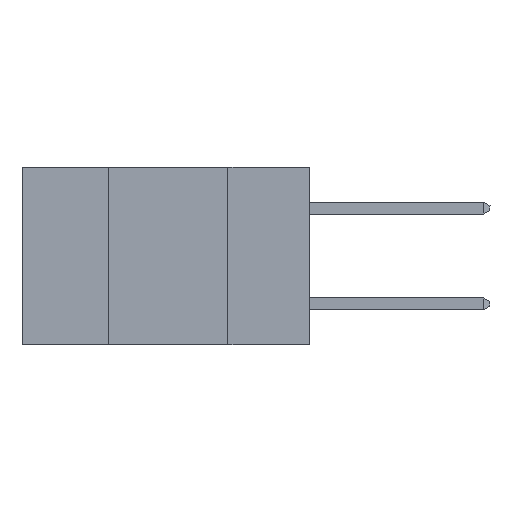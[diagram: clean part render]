
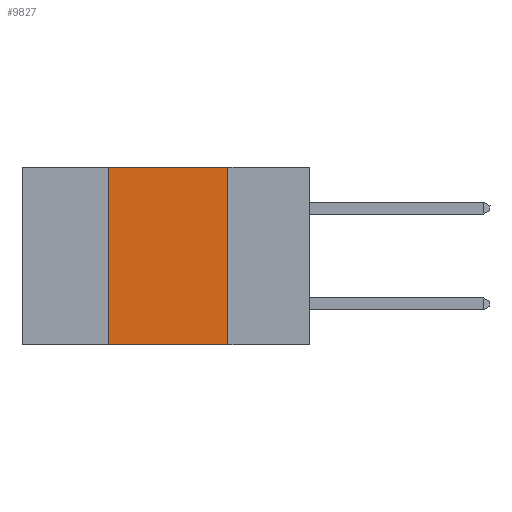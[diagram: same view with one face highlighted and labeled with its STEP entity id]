
A CAD part, left-side view. The second image highlights one B-rep face of the part: STEP entity #9827.
In plain terms, the highlighted planar face has unit normal (-1, 0, 0).
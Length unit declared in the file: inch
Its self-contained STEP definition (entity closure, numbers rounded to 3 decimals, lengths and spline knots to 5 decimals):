
#438 = FACE_OUTER_BOUND ( 'NONE', #6962, .T. ) ;
#467 = ORIENTED_EDGE ( 'NONE', *, *, #2694, .F. ) ;
#896 = CARTESIAN_POINT ( 'NONE',  ( 0., 0.42, 0. ) ) ;
#1671 = DIRECTION ( 'NONE',  ( 1., 0., 0. ) ) ;
#1912 = CARTESIAN_POINT ( 'NONE',  ( 0., 0.42, -0.37 ) ) ;
#2023 = VECTOR ( 'NONE', #8793, 39.37008 ) ;
#2311 = VERTEX_POINT ( 'NONE', #13477 ) ;
#2373 = CARTESIAN_POINT ( 'NONE',  ( 0., 0.6, 0. ) ) ;
#2694 = EDGE_CURVE ( 'NONE', #4705, #7857, #13482, .T. ) ;
#2707 = VECTOR ( 'NONE', #7215, 39.37008 ) ;
#3706 = EDGE_CURVE ( 'NONE', #7857, #2311, #12284, .T. ) ;
#4669 = CARTESIAN_POINT ( 'NONE',  ( 0., 0.6, -0.37 ) ) ;
#4705 = VERTEX_POINT ( 'NONE', #1912 ) ;
#4759 = VECTOR ( 'NONE', #16519, 39.37008 ) ;
#5038 = VECTOR ( 'NONE', #11826, 39.37008 ) ;
#5191 = LINE ( 'NONE', #5746, #4759 ) ;
#5746 = CARTESIAN_POINT ( 'NONE',  ( 0., 0.17, 0. ) ) ;
#6091 = EDGE_CURVE ( 'NONE', #4705, #11894, #9650, .T. ) ;
#6962 = EDGE_LOOP ( 'NONE', ( #15541, #15185, #467, #12990 ) ) ;
#7215 = DIRECTION ( 'NONE',  ( 0., 0., 1. ) ) ;
#7857 = VERTEX_POINT ( 'NONE', #896 ) ;
#8793 = DIRECTION ( 'NONE',  ( 0., -1., 0. ) ) ;
#9650 = LINE ( 'NONE', #4669, #2023 ) ;
#9779 = CARTESIAN_POINT ( 'NONE',  ( 0., 0.6, 0. ) ) ;
#9827 = ADVANCED_FACE ( 'NONE', ( #438 ), #16413, .F. ) ;
#9833 = CARTESIAN_POINT ( 'NONE',  ( 0., 0.17, -0.37 ) ) ;
#10840 = CARTESIAN_POINT ( 'NONE',  ( 0., 0.42, 0. ) ) ;
#11156 = DIRECTION ( 'NONE',  ( 0., 0., -1. ) ) ;
#11826 = DIRECTION ( 'NONE',  ( 0., -1., 0. ) ) ;
#11894 = VERTEX_POINT ( 'NONE', #9833 ) ;
#11906 = EDGE_CURVE ( 'NONE', #2311, #11894, #5191, .T. ) ;
#12284 = LINE ( 'NONE', #2373, #5038 ) ;
#12990 = ORIENTED_EDGE ( 'NONE', *, *, #6091, .T. ) ;
#13179 = AXIS2_PLACEMENT_3D ( 'NONE', #9779, #1671, #11156 ) ;
#13477 = CARTESIAN_POINT ( 'NONE',  ( 0., 0.17, 0. ) ) ;
#13482 = LINE ( 'NONE', #10840, #2707 ) ;
#15185 = ORIENTED_EDGE ( 'NONE', *, *, #3706, .F. ) ;
#15541 = ORIENTED_EDGE ( 'NONE', *, *, #11906, .F. ) ;
#16413 = PLANE ( 'NONE',  #13179 ) ;
#16519 = DIRECTION ( 'NONE',  ( 0., 0., -1. ) ) ;
